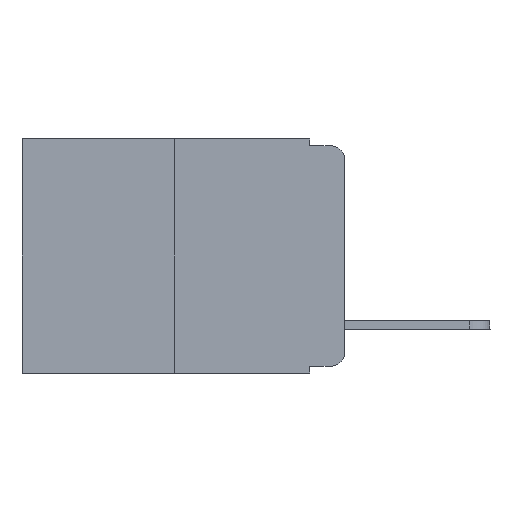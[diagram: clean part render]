
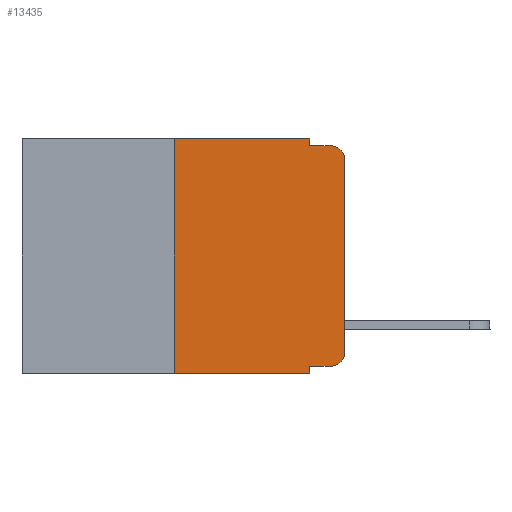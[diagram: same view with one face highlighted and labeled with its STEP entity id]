
A CAD part, left-side view. The second image highlights one B-rep face of the part: STEP entity #13435.
In plain terms, the highlighted planar face has unit normal (-1, 0, 0).
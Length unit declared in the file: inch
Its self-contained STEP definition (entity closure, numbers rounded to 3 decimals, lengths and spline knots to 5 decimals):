
#11 = CARTESIAN_POINT ( 'NONE',  ( 0., 0.25, -0.343 ) ) ;
#408 = ORIENTED_EDGE ( 'NONE', *, *, #14560, .T. ) ;
#858 = CARTESIAN_POINT ( 'NONE',  ( 0., 0.02, -0.313 ) ) ;
#936 = DIRECTION ( 'NONE',  ( 0., 0., 1. ) ) ;
#1060 = EDGE_CURVE ( 'NONE', #14346, #13723, #8986, .T. ) ;
#1139 = CARTESIAN_POINT ( 'NONE',  ( 0., 0.473, -0.343 ) ) ;
#1193 = VERTEX_POINT ( 'NONE', #8107 ) ;
#1195 = VERTEX_POINT ( 'NONE', #13389 ) ;
#1263 = CARTESIAN_POINT ( 'NONE',  ( 0., 0.051, -0.01 ) ) ;
#1268 = CARTESIAN_POINT ( 'NONE',  ( 0., 0.25, 0. ) ) ;
#1894 = DIRECTION ( 'NONE',  ( -1., 0., 0. ) ) ;
#1988 = CARTESIAN_POINT ( 'NONE',  ( 0., 0.473, 0. ) ) ;
#2157 = DIRECTION ( 'NONE',  ( 0., 0., -1. ) ) ;
#2185 = VERTEX_POINT ( 'NONE', #11 ) ;
#2222 = CARTESIAN_POINT ( 'NONE',  ( 0., 0.051, 0. ) ) ;
#2423 = CARTESIAN_POINT ( 'NONE',  ( 0., 0.051, 0. ) ) ;
#2498 = DIRECTION ( 'NONE',  ( 0., 0., -1. ) ) ;
#2722 = CARTESIAN_POINT ( 'NONE',  ( 0., 0.051, -0.333 ) ) ;
#2940 = CARTESIAN_POINT ( 'NONE',  ( 0., 0.051, -0.333 ) ) ;
#2969 = DIRECTION ( 'NONE',  ( 0., 0., 1. ) ) ;
#3007 = EDGE_CURVE ( 'NONE', #13496, #13932, #4801, .T. ) ;
#3090 = CIRCLE ( 'NONE', #4161, 0.02 ) ;
#3185 = DIRECTION ( 'NONE',  ( 0., -1., 0. ) ) ;
#3593 = DIRECTION ( 'NONE',  ( -1., 0., 0. ) ) ;
#3675 = EDGE_CURVE ( 'NONE', #15229, #13496, #14965, .T. ) ;
#3802 = EDGE_CURVE ( 'NONE', #14346, #16452, #10390, .T. ) ;
#3953 = CIRCLE ( 'NONE', #13565, 0.02 ) ;
#4017 = EDGE_CURVE ( 'NONE', #13932, #1195, #8267, .T. ) ;
#4113 = EDGE_CURVE ( 'NONE', #16452, #1193, #3090, .T. ) ;
#4149 = VECTOR ( 'NONE', #15484, 39.37008 ) ;
#4161 = AXIS2_PLACEMENT_3D ( 'NONE', #858, #1894, #7138 ) ;
#4801 = LINE ( 'NONE', #2222, #13006 ) ;
#4973 = CARTESIAN_POINT ( 'NONE',  ( 0., 0., -0.03 ) ) ;
#4997 = ORIENTED_EDGE ( 'NONE', *, *, #10100, .T. ) ;
#5161 = DIRECTION ( 'NONE',  ( 0., -1., 0. ) ) ;
#5406 = DIRECTION ( 'NONE',  ( 0., -1., 0. ) ) ;
#5483 = ORIENTED_EDGE ( 'NONE', *, *, #3802, .T. ) ;
#5543 = VECTOR ( 'NONE', #2969, 39.37008 ) ;
#6231 = VECTOR ( 'NONE', #3185, 39.37008 ) ;
#6666 = VECTOR ( 'NONE', #5406, 39.37008 ) ;
#6864 = ORIENTED_EDGE ( 'NONE', *, *, #4017, .F. ) ;
#7138 = DIRECTION ( 'NONE',  ( 0., 0., -1. ) ) ;
#8107 = CARTESIAN_POINT ( 'NONE',  ( 0., 0., -0.313 ) ) ;
#8267 = LINE ( 'NONE', #13463, #6666 ) ;
#8711 = PLANE ( 'NONE',  #16295 ) ;
#8977 = LINE ( 'NONE', #1139, #9135 ) ;
#8986 = LINE ( 'NONE', #2423, #9738 ) ;
#9135 = VECTOR ( 'NONE', #5161, 39.37008 ) ;
#9530 = LINE ( 'NONE', #14750, #5543 ) ;
#9738 = VECTOR ( 'NONE', #2498, 39.37008 ) ;
#9960 = CARTESIAN_POINT ( 'NONE',  ( 0., 0.25, 0. ) ) ;
#10061 = DIRECTION ( 'NONE',  ( 1., 0., 0. ) ) ;
#10100 = EDGE_CURVE ( 'NONE', #1193, #13355, #9530, .T. ) ;
#10390 = LINE ( 'NONE', #2722, #4149 ) ;
#10620 = EDGE_CURVE ( 'NONE', #2185, #13723, #8977, .T. ) ;
#11312 = EDGE_LOOP ( 'NONE', ( #4997, #408, #6864, #11721, #11727, #14968, #11432, #13090, #5483, #12442 ) ) ;
#11432 = ORIENTED_EDGE ( 'NONE', *, *, #10620, .T. ) ;
#11721 = ORIENTED_EDGE ( 'NONE', *, *, #3007, .F. ) ;
#11727 = ORIENTED_EDGE ( 'NONE', *, *, #3675, .F. ) ;
#12245 = CARTESIAN_POINT ( 'NONE',  ( 0., 0.02, -0.333 ) ) ;
#12442 = ORIENTED_EDGE ( 'NONE', *, *, #4113, .T. ) ;
#13006 = VECTOR ( 'NONE', #13815, 39.37008 ) ;
#13090 = ORIENTED_EDGE ( 'NONE', *, *, #1060, .F. ) ;
#13355 = VERTEX_POINT ( 'NONE', #4973 ) ;
#13389 = CARTESIAN_POINT ( 'NONE',  ( 0., 0.02, -0.01 ) ) ;
#13435 = ADVANCED_FACE ( 'NONE', ( #14080 ), #8711, .F. ) ;
#13463 = CARTESIAN_POINT ( 'NONE',  ( 0., 0.051, -0.01 ) ) ;
#13496 = VERTEX_POINT ( 'NONE', #14410 ) ;
#13565 = AXIS2_PLACEMENT_3D ( 'NONE', #14171, #3593, #2157 ) ;
#13672 = CARTESIAN_POINT ( 'NONE',  ( 0., 0.473, 0. ) ) ;
#13723 = VERTEX_POINT ( 'NONE', #14058 ) ;
#13815 = DIRECTION ( 'NONE',  ( 0., 0., -1. ) ) ;
#13932 = VERTEX_POINT ( 'NONE', #1263 ) ;
#14058 = CARTESIAN_POINT ( 'NONE',  ( 0., 0.051, -0.343 ) ) ;
#14080 = FACE_OUTER_BOUND ( 'NONE', #11312, .T. ) ;
#14171 = CARTESIAN_POINT ( 'NONE',  ( 0., 0.02, -0.03 ) ) ;
#14346 = VERTEX_POINT ( 'NONE', #2940 ) ;
#14410 = CARTESIAN_POINT ( 'NONE',  ( 0., 0.051, 0. ) ) ;
#14451 = VECTOR ( 'NONE', #936, 39.37008 ) ;
#14560 = EDGE_CURVE ( 'NONE', #13355, #1195, #3953, .T. ) ;
#14750 = CARTESIAN_POINT ( 'NONE',  ( 0., 0., 0. ) ) ;
#14965 = LINE ( 'NONE', #13672, #6231 ) ;
#14968 = ORIENTED_EDGE ( 'NONE', *, *, #16771, .F. ) ;
#15205 = LINE ( 'NONE', #9960, #14451 ) ;
#15229 = VERTEX_POINT ( 'NONE', #1268 ) ;
#15313 = DIRECTION ( 'NONE',  ( 0., 0., -1. ) ) ;
#15484 = DIRECTION ( 'NONE',  ( 0., -1., 0. ) ) ;
#16295 = AXIS2_PLACEMENT_3D ( 'NONE', #1988, #10061, #15313 ) ;
#16452 = VERTEX_POINT ( 'NONE', #12245 ) ;
#16771 = EDGE_CURVE ( 'NONE', #2185, #15229, #15205, .T. ) ;
